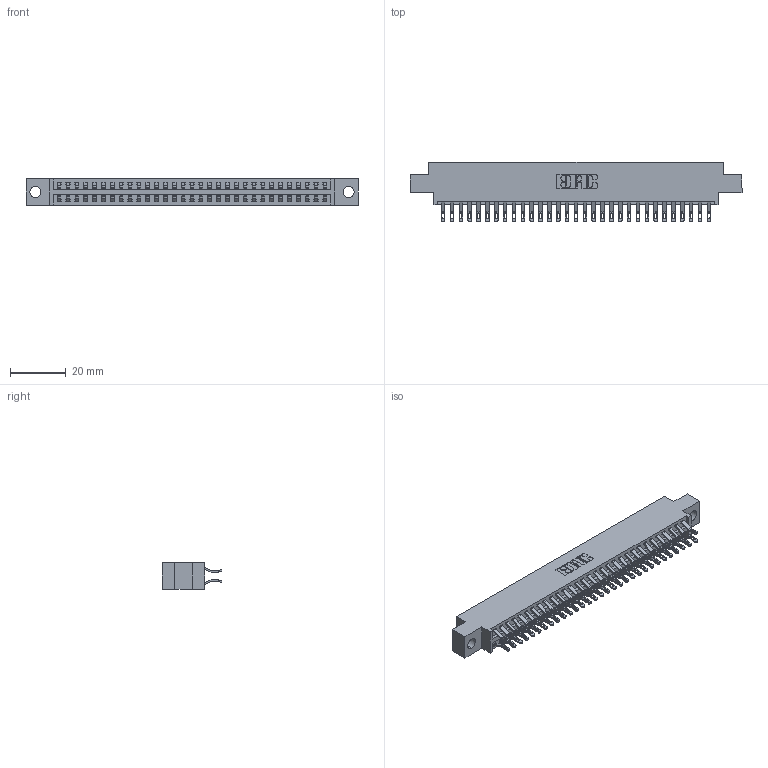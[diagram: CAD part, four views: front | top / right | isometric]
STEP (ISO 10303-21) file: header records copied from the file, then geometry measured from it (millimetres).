
FILE_DESCRIPTION (( 'STEP AP203' ), '1' );
FILE_NAME ('396-062-555-804.STEP', '2018-09-08T15:34:18', ( '' ), ( '' ), 'SwSTEP 2.0', 'SolidWorks 2016', '' );
FILE_SCHEMA (( 'CONFIG_CONTROL_DESIGN' ));
Length unit declared in the file: inch
Products named in the file (3): 346 Part_0.170 Offset - 0.156 Dia-TH; 345-292-001_555 Tail; 396-062-555-804
Assembly tree (63 placements, depth 2):
  396-062-555-804
    346 Part_0.170 Offset - 0.156 Dia-TH
    345-292-001_555 Tail  x62
Bounding box: 119 x 21.46 x 9.4 mm (x, y, z)
Volume: 11455.8 mm3; surface area: 16207.9 mm2
Topology: 63 solids, 63 shells, 3722 faces, 11687 edges, 7790 vertices
Faces by surface type: plane 2126, cylinder 1596
Entity records: 22173 total; most frequent: CARTESIAN_POINT 3706, ORIENTED_EDGE 3610, DIRECTION 3285, EDGE_CURVE 1805, LINE 1529, VECTOR 1529, VERTEX_POINT 1202, AXIS2_PLACEMENT_3D 878
